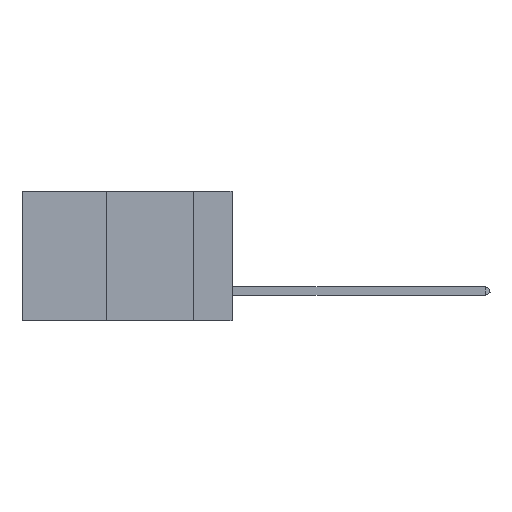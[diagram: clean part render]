
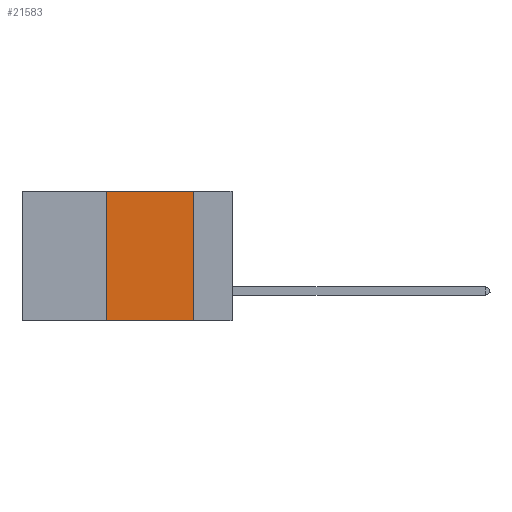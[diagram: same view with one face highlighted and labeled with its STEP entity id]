
A CAD part, left-side view. The second image highlights one B-rep face of the part: STEP entity #21583.
In plain terms, the highlighted planar face has unit normal (-1, 0, 0).
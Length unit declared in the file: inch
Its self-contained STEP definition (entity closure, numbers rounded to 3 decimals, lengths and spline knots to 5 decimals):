
#448 = CARTESIAN_POINT ( 'NONE',  ( 0., 0.6, -0.37 ) ) ;
#1244 = LINE ( 'NONE', #32713, #8314 ) ;
#1653 = FACE_OUTER_BOUND ( 'NONE', #43896, .T. ) ;
#3379 = VECTOR ( 'NONE', #21269, 39.37008 ) ;
#4452 = ORIENTED_EDGE ( 'NONE', *, *, #31873, .T. ) ;
#4802 = EDGE_CURVE ( 'NONE', #31511, #35158, #29120, .T. ) ;
#7142 = CARTESIAN_POINT ( 'NONE',  ( 0., 0.6, 0. ) ) ;
#8231 = VECTOR ( 'NONE', #19531, 39.37008 ) ;
#8314 = VECTOR ( 'NONE', #11207, 39.37008 ) ;
#10302 = LINE ( 'NONE', #15450, #21812 ) ;
#10485 = LINE ( 'NONE', #448, #3379 ) ;
#11207 = DIRECTION ( 'NONE',  ( 0., 0., 1. ) ) ;
#12996 = CARTESIAN_POINT ( 'NONE',  ( 0., 0.36, 0. ) ) ;
#13370 = ORIENTED_EDGE ( 'NONE', *, *, #25906, .F. ) ;
#13486 = VERTEX_POINT ( 'NONE', #12996 ) ;
#15450 = CARTESIAN_POINT ( 'NONE',  ( 0., 0.6, 0. ) ) ;
#15741 = DIRECTION ( 'NONE',  ( 0., -1., 0. ) ) ;
#16849 = AXIS2_PLACEMENT_3D ( 'NONE', #7142, #35197, #42213 ) ;
#19531 = DIRECTION ( 'NONE',  ( 0., 0., -1. ) ) ;
#20546 = EDGE_CURVE ( 'NONE', #23869, #13486, #1244, .T. ) ;
#21269 = DIRECTION ( 'NONE',  ( 0., -1., 0. ) ) ;
#21409 = PLANE ( 'NONE',  #16849 ) ;
#21583 = ADVANCED_FACE ( 'NONE', ( #1653 ), #21409, .F. ) ;
#21812 = VECTOR ( 'NONE', #15741, 39.37008 ) ;
#23869 = VERTEX_POINT ( 'NONE', #36686 ) ;
#25906 = EDGE_CURVE ( 'NONE', #13486, #31511, #10302, .T. ) ;
#26145 = CARTESIAN_POINT ( 'NONE',  ( 0., 0.11, 0. ) ) ;
#29120 = LINE ( 'NONE', #26145, #8231 ) ;
#31511 = VERTEX_POINT ( 'NONE', #43448 ) ;
#31873 = EDGE_CURVE ( 'NONE', #23869, #35158, #10485, .T. ) ;
#32713 = CARTESIAN_POINT ( 'NONE',  ( 0., 0.36, 0. ) ) ;
#35158 = VERTEX_POINT ( 'NONE', #39477 ) ;
#35197 = DIRECTION ( 'NONE',  ( 1., 0., 0. ) ) ;
#36686 = CARTESIAN_POINT ( 'NONE',  ( 0., 0.36, -0.37 ) ) ;
#38502 = ORIENTED_EDGE ( 'NONE', *, *, #20546, .F. ) ;
#39477 = CARTESIAN_POINT ( 'NONE',  ( 0., 0.11, -0.37 ) ) ;
#40250 = ORIENTED_EDGE ( 'NONE', *, *, #4802, .F. ) ;
#42213 = DIRECTION ( 'NONE',  ( 0., 0., -1. ) ) ;
#43448 = CARTESIAN_POINT ( 'NONE',  ( 0., 0.11, 0. ) ) ;
#43896 = EDGE_LOOP ( 'NONE', ( #40250, #13370, #38502, #4452 ) ) ;
